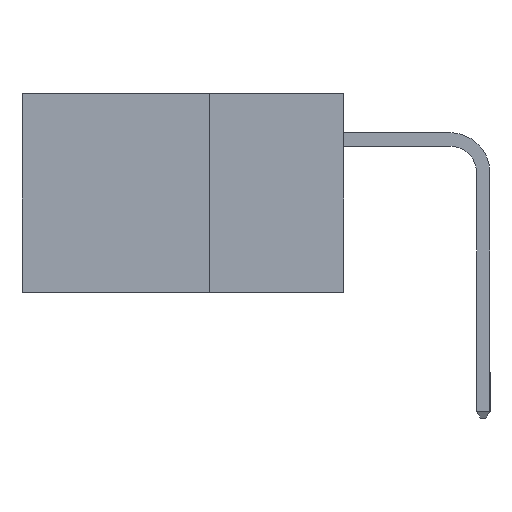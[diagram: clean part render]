
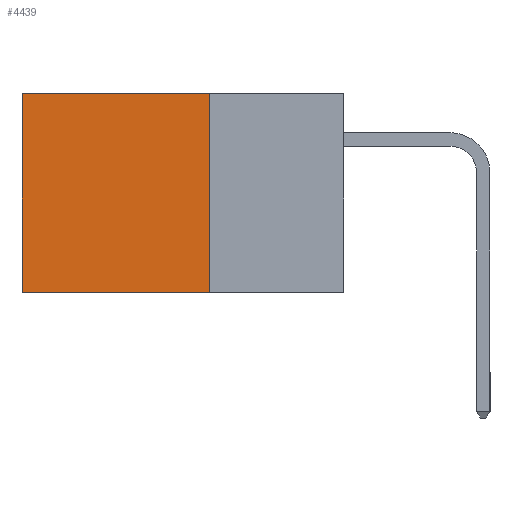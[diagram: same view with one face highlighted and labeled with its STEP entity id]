
A CAD part, left-side view. The second image highlights one B-rep face of the part: STEP entity #4439.
In plain terms, the highlighted planar face has unit normal (-1, 0, 0).
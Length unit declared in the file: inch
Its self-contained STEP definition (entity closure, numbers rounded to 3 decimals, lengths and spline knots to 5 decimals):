
#602 = LINE ( 'NONE', #2160, #12919 ) ;
#1272 = CARTESIAN_POINT ( 'NONE',  ( 0.298, 0.25, -0.37 ) ) ;
#1297 = VECTOR ( 'NONE', #11492, 39.37008 ) ;
#1337 = ORIENTED_EDGE ( 'NONE', *, *, #1894, .T. ) ;
#1820 = DIRECTION ( 'NONE',  ( 1., 0., 0. ) ) ;
#1894 = EDGE_CURVE ( 'NONE', #8403, #12598, #602, .T. ) ;
#2160 = CARTESIAN_POINT ( 'NONE',  ( 0.298, 0.6, 0. ) ) ;
#2318 = DIRECTION ( 'NONE',  ( 0., 1., 0. ) ) ;
#2383 = DIRECTION ( 'NONE',  ( 0., 0., -1. ) ) ;
#2534 = VECTOR ( 'NONE', #2318, 39.37008 ) ;
#2651 = EDGE_CURVE ( 'NONE', #14767, #12598, #9264, .T. ) ;
#4331 = EDGE_CURVE ( 'NONE', #7733, #8403, #14987, .T. ) ;
#4439 = ADVANCED_FACE ( 'NONE', ( #13244 ), #13654, .F. ) ;
#4662 = ORIENTED_EDGE ( 'NONE', *, *, #7598, .F. ) ;
#5906 = AXIS2_PLACEMENT_3D ( 'NONE', #10250, #1820, #7753 ) ;
#6570 = EDGE_LOOP ( 'NONE', ( #1337, #6924, #4662, #6927 ) ) ;
#6605 = CARTESIAN_POINT ( 'NONE',  ( 0.298, 0.6, -0.37 ) ) ;
#6924 = ORIENTED_EDGE ( 'NONE', *, *, #2651, .F. ) ;
#6927 = ORIENTED_EDGE ( 'NONE', *, *, #4331, .T. ) ;
#7598 = EDGE_CURVE ( 'NONE', #7733, #14767, #10032, .T. ) ;
#7733 = VERTEX_POINT ( 'NONE', #8431 ) ;
#7753 = DIRECTION ( 'NONE',  ( 0., 0., -1. ) ) ;
#8403 = VERTEX_POINT ( 'NONE', #10277 ) ;
#8431 = CARTESIAN_POINT ( 'NONE',  ( 0.298, 0.25, 0. ) ) ;
#9264 = LINE ( 'NONE', #13332, #2534 ) ;
#9973 = CARTESIAN_POINT ( 'NONE',  ( 0.298, 0.25, 0. ) ) ;
#10032 = LINE ( 'NONE', #13445, #14873 ) ;
#10250 = CARTESIAN_POINT ( 'NONE',  ( 0.298, 0.25, 0. ) ) ;
#10277 = CARTESIAN_POINT ( 'NONE',  ( 0.298, 0.6, 0. ) ) ;
#11492 = DIRECTION ( 'NONE',  ( 0., 1., 0. ) ) ;
#12598 = VERTEX_POINT ( 'NONE', #6605 ) ;
#12919 = VECTOR ( 'NONE', #15620, 39.37008 ) ;
#13244 = FACE_OUTER_BOUND ( 'NONE', #6570, .T. ) ;
#13332 = CARTESIAN_POINT ( 'NONE',  ( 0.298, 0.25, -0.37 ) ) ;
#13445 = CARTESIAN_POINT ( 'NONE',  ( 0.298, 0.25, 0. ) ) ;
#13654 = PLANE ( 'NONE',  #5906 ) ;
#14767 = VERTEX_POINT ( 'NONE', #1272 ) ;
#14873 = VECTOR ( 'NONE', #2383, 39.37008 ) ;
#14987 = LINE ( 'NONE', #9973, #1297 ) ;
#15620 = DIRECTION ( 'NONE',  ( 0., 0., -1. ) ) ;
